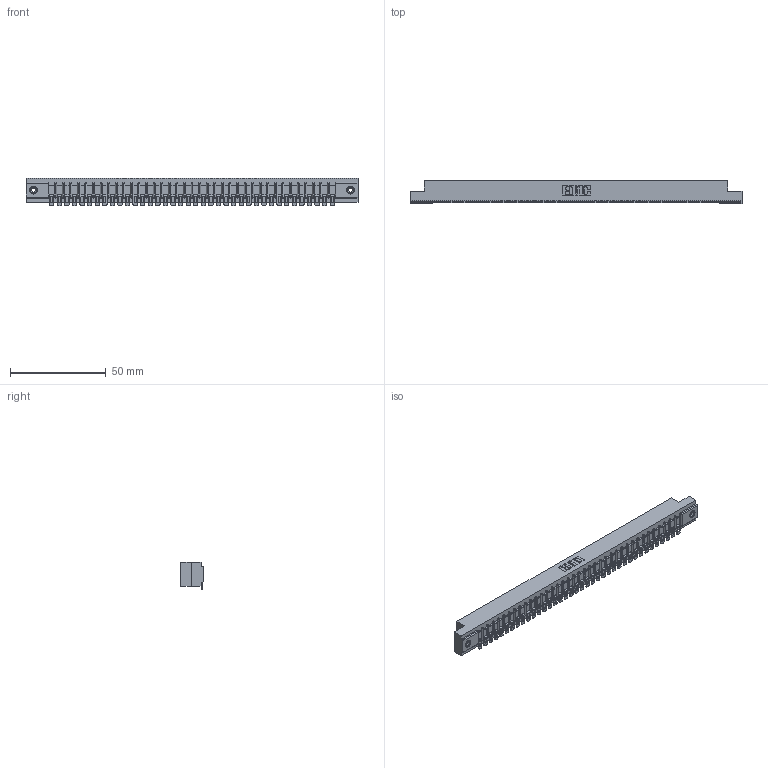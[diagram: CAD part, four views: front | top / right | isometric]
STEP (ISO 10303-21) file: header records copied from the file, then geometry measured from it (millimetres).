
FILE_DESCRIPTION (( 'STEP AP203' ), '1' );
FILE_NAME ('307-038-454-108.STEP', '2020-09-29T06:38:12', ( '' ), ( '' ), 'SwSTEP 2.0', 'SolidWorks 2020', '' );
FILE_SCHEMA (( 'CONFIG_CONTROL_DESIGN' ));
Length unit declared in the file: inch
Products named in the file (4): 307 Part_.156 Dia Mounting Holes; 345-250-001_345-250-003-102; 307-038-454-108; 307-290-002_554
Assembly tree (41 placements, depth 2):
  307-038-454-108
    307 Part_.156 Dia Mounting Holes
    307-290-002_554  x38
    345-250-001_345-250-003-102  x2
Bounding box: 173.58 x 12.01 x 14.52 mm (x, y, z)
Volume: 18553 mm3; surface area: 23406.1 mm2
Topology: 41 solids, 41 shells, 3295 faces, 10073 edges, 6602 vertices
Faces by surface type: plane 1850, cylinder 1351, sphere 78, cone 12, torus 4
Entity records: 35220 total; most frequent: CARTESIAN_POINT 5921, ORIENTED_EDGE 5904, DIRECTION 5770, EDGE_CURVE 2952, VECTOR 2252, LINE 2252, VERTEX_POINT 1910, AXIS2_PLACEMENT_3D 1759
